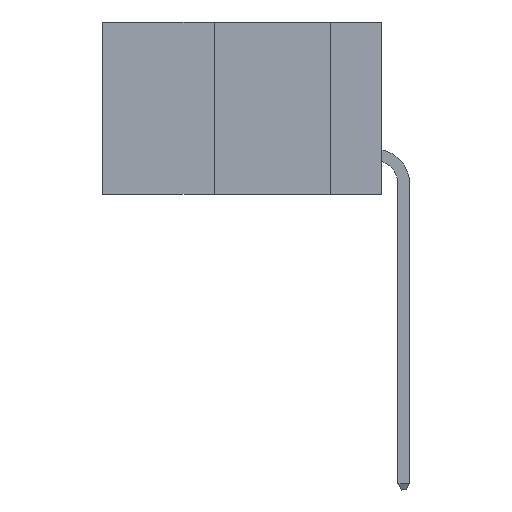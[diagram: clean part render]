
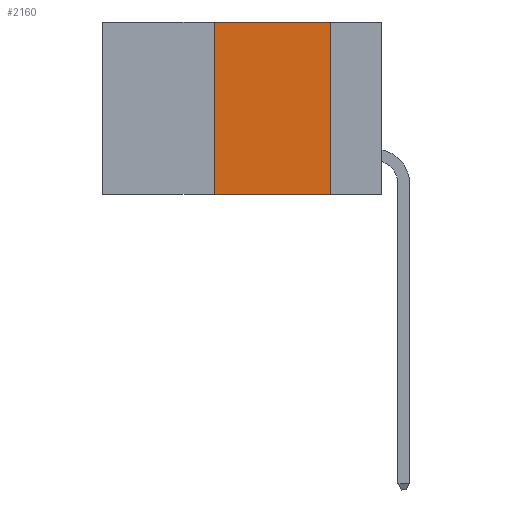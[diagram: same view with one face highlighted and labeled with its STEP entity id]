
A CAD part, left-side view. The second image highlights one B-rep face of the part: STEP entity #2160.
In plain terms, the highlighted planar face has unit normal (-1, 0, 0).
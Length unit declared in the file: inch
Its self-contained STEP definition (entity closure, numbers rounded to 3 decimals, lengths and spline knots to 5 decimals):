
#153 = EDGE_LOOP ( 'NONE', ( #14110, #8617, #10284, #12000 ) ) ;
#301 = DIRECTION ( 'NONE',  ( 0., -1., 0. ) ) ;
#1063 = CARTESIAN_POINT ( 'NONE',  ( 0., 0.36, 0. ) ) ;
#1437 = DIRECTION ( 'NONE',  ( 0., 0., 1. ) ) ;
#1824 = CARTESIAN_POINT ( 'NONE',  ( 0., 0.6, 0. ) ) ;
#2016 = FACE_OUTER_BOUND ( 'NONE', #153, .T. ) ;
#2160 = ADVANCED_FACE ( 'NONE', ( #2016 ), #5084, .F. ) ;
#2943 = EDGE_CURVE ( 'NONE', #9763, #6861, #6538, .T. ) ;
#3048 = DIRECTION ( 'NONE',  ( 0., -1., 0. ) ) ;
#3443 = VECTOR ( 'NONE', #301, 39.37008 ) ;
#3605 = AXIS2_PLACEMENT_3D ( 'NONE', #1824, #12863, #6183 ) ;
#4126 = LINE ( 'NONE', #7096, #14414 ) ;
#4557 = EDGE_CURVE ( 'NONE', #5636, #6202, #4126, .T. ) ;
#4935 = VECTOR ( 'NONE', #3048, 39.37008 ) ;
#5084 = PLANE ( 'NONE',  #3605 ) ;
#5223 = LINE ( 'NONE', #13580, #3443 ) ;
#5593 = CARTESIAN_POINT ( 'NONE',  ( 0., 0.11, 0. ) ) ;
#5636 = VERTEX_POINT ( 'NONE', #14329 ) ;
#6183 = DIRECTION ( 'NONE',  ( 0., 0., -1. ) ) ;
#6202 = VERTEX_POINT ( 'NONE', #1063 ) ;
#6538 = LINE ( 'NONE', #12948, #11226 ) ;
#6861 = VERTEX_POINT ( 'NONE', #7680 ) ;
#7096 = CARTESIAN_POINT ( 'NONE',  ( 0., 0.36, 0. ) ) ;
#7680 = CARTESIAN_POINT ( 'NONE',  ( 0., 0.11, -0.37 ) ) ;
#8617 = ORIENTED_EDGE ( 'NONE', *, *, #13522, .F. ) ;
#9669 = DIRECTION ( 'NONE',  ( 0., 0., -1. ) ) ;
#9763 = VERTEX_POINT ( 'NONE', #5593 ) ;
#10284 = ORIENTED_EDGE ( 'NONE', *, *, #4557, .F. ) ;
#11226 = VECTOR ( 'NONE', #9669, 39.37008 ) ;
#11531 = CARTESIAN_POINT ( 'NONE',  ( 0., 0.6, -0.37 ) ) ;
#12000 = ORIENTED_EDGE ( 'NONE', *, *, #12025, .T. ) ;
#12025 = EDGE_CURVE ( 'NONE', #5636, #6861, #12410, .T. ) ;
#12410 = LINE ( 'NONE', #11531, #4935 ) ;
#12863 = DIRECTION ( 'NONE',  ( 1., 0., 0. ) ) ;
#12948 = CARTESIAN_POINT ( 'NONE',  ( 0., 0.11, 0. ) ) ;
#13522 = EDGE_CURVE ( 'NONE', #6202, #9763, #5223, .T. ) ;
#13580 = CARTESIAN_POINT ( 'NONE',  ( 0., 0.6, 0. ) ) ;
#14110 = ORIENTED_EDGE ( 'NONE', *, *, #2943, .F. ) ;
#14329 = CARTESIAN_POINT ( 'NONE',  ( 0., 0.36, -0.37 ) ) ;
#14414 = VECTOR ( 'NONE', #1437, 39.37008 ) ;
